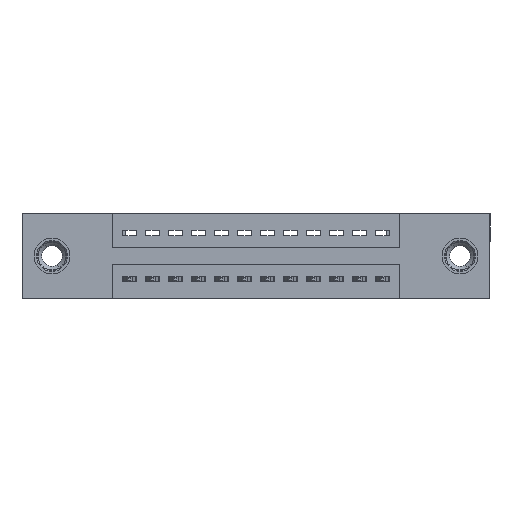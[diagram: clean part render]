
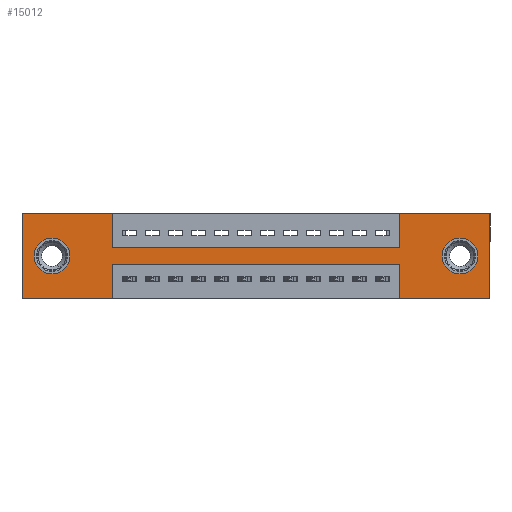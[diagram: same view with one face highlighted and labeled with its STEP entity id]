
A CAD part, front view. The second image highlights one B-rep face of the part: STEP entity #15012.
In plain terms, the highlighted planar face has unit normal (0, -1, 0).
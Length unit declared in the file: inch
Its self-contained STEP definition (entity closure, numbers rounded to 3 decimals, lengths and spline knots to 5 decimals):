
#67 = VERTEX_POINT ( 'NONE', #13272 ) ;
#251 = DIRECTION ( 'NONE',  ( 0., 0., 1. ) ) ;
#388 = ORIENTED_EDGE ( 'NONE', *, *, #7118, .F. ) ;
#1035 = CARTESIAN_POINT ( 'NONE',  ( 0.3925, 0., -0.15 ) ) ;
#1115 = ORIENTED_EDGE ( 'NONE', *, *, #4501, .F. ) ;
#1186 = CARTESIAN_POINT ( 'NONE',  ( 1.905, 0., -0.107 ) ) ;
#1192 = VERTEX_POINT ( 'NONE', #11312 ) ;
#1231 = VERTEX_POINT ( 'NONE', #5958 ) ;
#1251 = ORIENTED_EDGE ( 'NONE', *, *, #8263, .T. ) ;
#1778 = CARTESIAN_POINT ( 'NONE',  ( 1.6425, 0., -0.37 ) ) ;
#1843 = VERTEX_POINT ( 'NONE', #16408 ) ;
#1845 = EDGE_LOOP ( 'NONE', ( #6718, #1251 ) ) ;
#2029 = CARTESIAN_POINT ( 'NONE',  ( 2.035, 0., 0. ) ) ;
#2034 = CARTESIAN_POINT ( 'NONE',  ( 0., 0., 0. ) ) ;
#2136 = CARTESIAN_POINT ( 'NONE',  ( 1.905, 0., -0.185 ) ) ;
#2154 = CARTESIAN_POINT ( 'NONE',  ( 1.6425, 0., 0. ) ) ;
#2187 = LINE ( 'NONE', #16552, #16467 ) ;
#2367 = DIRECTION ( 'NONE',  ( 0., 0., -1. ) ) ;
#2391 = LINE ( 'NONE', #10585, #16845 ) ;
#2892 = DIRECTION ( 'NONE',  ( 0., 1., 0. ) ) ;
#2987 = CARTESIAN_POINT ( 'NONE',  ( 0.3925, 0., 0. ) ) ;
#3324 = EDGE_CURVE ( 'NONE', #1843, #13675, #16887, .T. ) ;
#3459 = VECTOR ( 'NONE', #17659, 39.37008 ) ;
#3482 = DIRECTION ( 'NONE',  ( -1., 0., 0. ) ) ;
#3567 = DIRECTION ( 'NONE',  ( 0., 0., -1. ) ) ;
#3885 = CARTESIAN_POINT ( 'NONE',  ( 2.035, 0., 0. ) ) ;
#3927 = DIRECTION ( 'NONE',  ( 0., 1., 0. ) ) ;
#4107 = ORIENTED_EDGE ( 'NONE', *, *, #14035, .F. ) ;
#4133 = ORIENTED_EDGE ( 'NONE', *, *, #17393, .F. ) ;
#4180 = DIRECTION ( 'NONE',  ( 0., 0., 1. ) ) ;
#4194 = ORIENTED_EDGE ( 'NONE', *, *, #5025, .F. ) ;
#4438 = EDGE_LOOP ( 'NONE', ( #5813, #17188 ) ) ;
#4440 = CARTESIAN_POINT ( 'NONE',  ( 0.13, 0., -0.107 ) ) ;
#4501 = EDGE_CURVE ( 'NONE', #6955, #1843, #7126, .T. ) ;
#4890 = CARTESIAN_POINT ( 'NONE',  ( 0.3925, 0., -0.22 ) ) ;
#5025 = EDGE_CURVE ( 'NONE', #13675, #15396, #2391, .T. ) ;
#5035 = DIRECTION ( 'NONE',  ( 1., 0., 0. ) ) ;
#5065 = DIRECTION ( 'NONE',  ( 0., -1., 0. ) ) ;
#5343 = AXIS2_PLACEMENT_3D ( 'NONE', #2136, #13107, #3567 ) ;
#5643 = VERTEX_POINT ( 'NONE', #13249 ) ;
#5813 = ORIENTED_EDGE ( 'NONE', *, *, #8482, .T. ) ;
#5862 = FACE_BOUND ( 'NONE', #4438, .T. ) ;
#5958 = CARTESIAN_POINT ( 'NONE',  ( 1.905, 0., -0.263 ) ) ;
#5960 = DIRECTION ( 'NONE',  ( 0., 0., 1. ) ) ;
#6124 = CARTESIAN_POINT ( 'NONE',  ( 1.6425, 0., 0. ) ) ;
#6550 = DIRECTION ( 'NONE',  ( 0., 0., -1. ) ) ;
#6718 = ORIENTED_EDGE ( 'NONE', *, *, #14245, .T. ) ;
#6955 = VERTEX_POINT ( 'NONE', #8636 ) ;
#7081 = AXIS2_PLACEMENT_3D ( 'NONE', #12348, #2892, #4180 ) ;
#7118 = EDGE_CURVE ( 'NONE', #5643, #8435, #12113, .T. ) ;
#7126 = LINE ( 'NONE', #1035, #3459 ) ;
#7403 = ORIENTED_EDGE ( 'NONE', *, *, #11248, .F. ) ;
#7597 = ORIENTED_EDGE ( 'NONE', *, *, #17702, .F. ) ;
#7651 = CARTESIAN_POINT ( 'NONE',  ( 0., 0., 0. ) ) ;
#7666 = LINE ( 'NONE', #11786, #16935 ) ;
#7768 = DIRECTION ( 'NONE',  ( 0., 0., 1. ) ) ;
#7852 = FACE_OUTER_BOUND ( 'NONE', #7855, .T. ) ;
#7855 = EDGE_LOOP ( 'NONE', ( #4133, #12261, #7403, #10702, #17336, #4194, #15444, #1115, #7597, #388, #4107, #17025 ) ) ;
#8263 = EDGE_CURVE ( 'NONE', #1231, #12608, #14866, .T. ) ;
#8306 = CIRCLE ( 'NONE', #13254, 0.078 ) ;
#8435 = VERTEX_POINT ( 'NONE', #12288 ) ;
#8482 = EDGE_CURVE ( 'NONE', #9155, #12966, #16406, .T. ) ;
#8540 = VERTEX_POINT ( 'NONE', #9091 ) ;
#8636 = CARTESIAN_POINT ( 'NONE',  ( 0.3925, 0., -0.15 ) ) ;
#9091 = CARTESIAN_POINT ( 'NONE',  ( 1.6425, 0., -0.37 ) ) ;
#9155 = VERTEX_POINT ( 'NONE', #4440 ) ;
#9157 = VECTOR ( 'NONE', #5960, 39.37008 ) ;
#9490 = CARTESIAN_POINT ( 'NONE',  ( 0.3925, 0., -0.37 ) ) ;
#10041 = CARTESIAN_POINT ( 'NONE',  ( 0., 0., -0.37 ) ) ;
#10101 = DIRECTION ( 'NONE',  ( -1., 0., 0. ) ) ;
#10193 = LINE ( 'NONE', #10041, #13228 ) ;
#10242 = LINE ( 'NONE', #7651, #14331 ) ;
#10366 = CARTESIAN_POINT ( 'NONE',  ( 0., 0., -0.37 ) ) ;
#10461 = EDGE_CURVE ( 'NONE', #1192, #67, #7666, .T. ) ;
#10540 = DIRECTION ( 'NONE',  ( 1., 0., 0. ) ) ;
#10585 = CARTESIAN_POINT ( 'NONE',  ( 0., 0., 0. ) ) ;
#10589 = LINE ( 'NONE', #2987, #15774 ) ;
#10636 = EDGE_CURVE ( 'NONE', #12966, #9155, #12003, .T. ) ;
#10702 = ORIENTED_EDGE ( 'NONE', *, *, #12170, .F. ) ;
#10897 = LINE ( 'NONE', #3885, #15879 ) ;
#10968 = DIRECTION ( 'NONE',  ( -1., 0., 0. ) ) ;
#11248 = EDGE_CURVE ( 'NONE', #8540, #12188, #13014, .T. ) ;
#11312 = CARTESIAN_POINT ( 'NONE',  ( 0.3925, 0., -0.37 ) ) ;
#11483 = EDGE_CURVE ( 'NONE', #15396, #15100, #10897, .T. ) ;
#11642 = DIRECTION ( 'NONE',  ( 0., 0., 1. ) ) ;
#11786 = CARTESIAN_POINT ( 'NONE',  ( 0., 0., -0.37 ) ) ;
#12003 = CIRCLE ( 'NONE', #16936, 0.078 ) ;
#12045 = DIRECTION ( 'NONE',  ( 0., 0., -1. ) ) ;
#12113 = LINE ( 'NONE', #2034, #16645 ) ;
#12170 = EDGE_CURVE ( 'NONE', #15100, #8540, #10193, .T. ) ;
#12188 = VERTEX_POINT ( 'NONE', #13001 ) ;
#12261 = ORIENTED_EDGE ( 'NONE', *, *, #16799, .F. ) ;
#12288 = CARTESIAN_POINT ( 'NONE',  ( 0.3925, 0., 0. ) ) ;
#12348 = CARTESIAN_POINT ( 'NONE',  ( 0.13, 0., -0.185 ) ) ;
#12608 = VERTEX_POINT ( 'NONE', #1186 ) ;
#12966 = VERTEX_POINT ( 'NONE', #16461 ) ;
#13001 = CARTESIAN_POINT ( 'NONE',  ( 1.6425, 0., -0.22 ) ) ;
#13003 = FACE_BOUND ( 'NONE', #1845, .T. ) ;
#13014 = LINE ( 'NONE', #1778, #9157 ) ;
#13107 = DIRECTION ( 'NONE',  ( 0., 1., 0. ) ) ;
#13228 = VECTOR ( 'NONE', #10101, 39.37008 ) ;
#13249 = CARTESIAN_POINT ( 'NONE',  ( 0., 0., 0. ) ) ;
#13254 = AXIS2_PLACEMENT_3D ( 'NONE', #13456, #3927, #12045 ) ;
#13272 = CARTESIAN_POINT ( 'NONE',  ( 0., 0., -0.37 ) ) ;
#13386 = VECTOR ( 'NONE', #2367, 39.37008 ) ;
#13456 = CARTESIAN_POINT ( 'NONE',  ( 1.905, 0., -0.185 ) ) ;
#13675 = VERTEX_POINT ( 'NONE', #6124 ) ;
#13822 = LINE ( 'NONE', #9490, #13386 ) ;
#13887 = VERTEX_POINT ( 'NONE', #4890 ) ;
#14035 = EDGE_CURVE ( 'NONE', #67, #5643, #10242, .T. ) ;
#14245 = EDGE_CURVE ( 'NONE', #12608, #1231, #8306, .T. ) ;
#14331 = VECTOR ( 'NONE', #7768, 39.37008 ) ;
#14454 = PLANE ( 'NONE',  #16224 ) ;
#14866 = CIRCLE ( 'NONE', #5343, 0.078 ) ;
#14988 = DIRECTION ( 'NONE',  ( 0., 0., -1. ) ) ;
#15012 = ADVANCED_FACE ( 'NONE', ( #13003, #5862, #7852 ), #14454, .T. ) ;
#15100 = VERTEX_POINT ( 'NONE', #17665 ) ;
#15321 = CARTESIAN_POINT ( 'NONE',  ( 0.13, 0., -0.185 ) ) ;
#15396 = VERTEX_POINT ( 'NONE', #2029 ) ;
#15444 = ORIENTED_EDGE ( 'NONE', *, *, #3324, .F. ) ;
#15464 = DIRECTION ( 'NONE',  ( 0., 0., -1. ) ) ;
#15774 = VECTOR ( 'NONE', #15464, 39.37008 ) ;
#15879 = VECTOR ( 'NONE', #14988, 39.37008 ) ;
#16073 = VECTOR ( 'NONE', #11642, 39.37008 ) ;
#16224 = AXIS2_PLACEMENT_3D ( 'NONE', #10366, #5065, #6550 ) ;
#16406 = CIRCLE ( 'NONE', #7081, 0.078 ) ;
#16408 = CARTESIAN_POINT ( 'NONE',  ( 1.6425, 0., -0.15 ) ) ;
#16461 = CARTESIAN_POINT ( 'NONE',  ( 0.13, 0., -0.263 ) ) ;
#16467 = VECTOR ( 'NONE', #10968, 39.37008 ) ;
#16552 = CARTESIAN_POINT ( 'NONE',  ( 0.3925, 0., -0.22 ) ) ;
#16645 = VECTOR ( 'NONE', #10540, 39.37008 ) ;
#16713 = DIRECTION ( 'NONE',  ( 0., 1., 0. ) ) ;
#16799 = EDGE_CURVE ( 'NONE', #12188, #13887, #2187, .T. ) ;
#16845 = VECTOR ( 'NONE', #5035, 39.37008 ) ;
#16887 = LINE ( 'NONE', #2154, #16073 ) ;
#16935 = VECTOR ( 'NONE', #3482, 39.37008 ) ;
#16936 = AXIS2_PLACEMENT_3D ( 'NONE', #15321, #16713, #251 ) ;
#17025 = ORIENTED_EDGE ( 'NONE', *, *, #10461, .F. ) ;
#17188 = ORIENTED_EDGE ( 'NONE', *, *, #10636, .T. ) ;
#17336 = ORIENTED_EDGE ( 'NONE', *, *, #11483, .F. ) ;
#17393 = EDGE_CURVE ( 'NONE', #13887, #1192, #13822, .T. ) ;
#17659 = DIRECTION ( 'NONE',  ( 1., 0., 0. ) ) ;
#17665 = CARTESIAN_POINT ( 'NONE',  ( 2.035, 0., -0.37 ) ) ;
#17702 = EDGE_CURVE ( 'NONE', #8435, #6955, #10589, .T. ) ;
